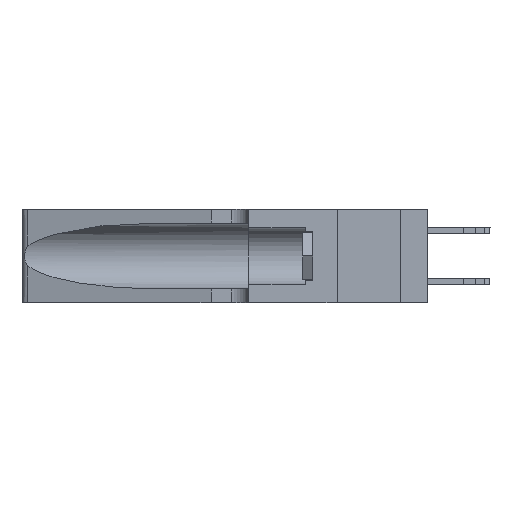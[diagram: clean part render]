
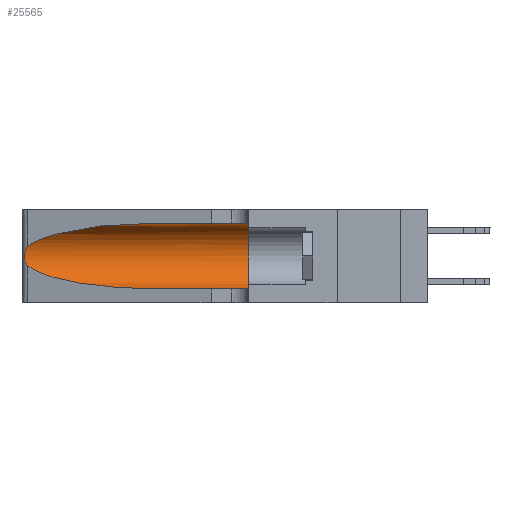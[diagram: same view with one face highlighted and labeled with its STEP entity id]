
A CAD part, left-side view. The second image highlights one B-rep face of the part: STEP entity #25565.
In plain terms, the highlighted cylindrical face has radius 3.308 mm (diameter 6.617 mm), a partial arc.
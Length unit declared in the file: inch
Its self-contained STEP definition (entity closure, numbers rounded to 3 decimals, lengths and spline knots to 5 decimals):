
#877 = CARTESIAN_POINT ( 'NONE',  ( 0.2373, 1.15595, 0.08982 ) ) ;
#1038 = ORIENTED_EDGE ( 'NONE', *, *, #34317, .F. ) ;
#1173 = DIRECTION ( 'NONE',  ( 0., 1., 0. ) ) ;
#3045 = CARTESIAN_POINT ( 'NONE',  ( 0.25787, 1.23484, 0.2124 ) ) ;
#4140 = DIRECTION ( 'NONE',  ( 0., -1., 0. ) ) ;
#4218 = DIRECTION ( 'NONE',  ( 0., 0., 1. ) ) ;
#6433 = B_SPLINE_CURVE_WITH_KNOTS ( 'NONE', 3,
 ( #35911, #26943, #24569, #3045, #27586, #21166, #18249, #9301, #9547, #6499, #30630, #33368, #12168, #15463 ),
 .UNSPECIFIED., .F., .F.,
 ( 4, 2, 2, 2, 2, 2, 4 ),
 ( 0., 0.00027, 0.00053, 0.00107, 0.0016, 0.00187, 0.00214 ),
 .UNSPECIFIED. ) ;
#6499 = CARTESIAN_POINT ( 'NONE',  ( 0.25856, 1.23593, 0.16098 ) ) ;
#6806 = CARTESIAN_POINT ( 'NONE',  ( 0.1305, 1.61858, 0.185 ) ) ;
#7029 = CYLINDRICAL_SURFACE ( 'NONE', #19081, 0.13025 ) ;
#9301 = CARTESIAN_POINT ( 'NONE',  ( 0.26075, 1.23896, 0.178 ) ) ;
#9453 = LINE ( 'NONE', #23665, #11319 ) ;
#9547 = CARTESIAN_POINT ( 'NONE',  ( 0.26017, 1.23833, 0.17102 ) ) ;
#10111 = CARTESIAN_POINT ( 'NONE',  ( 0.25487, 1.22718, 0.22369 ) ) ;
#10358 = CARTESIAN_POINT ( 'NONE',  ( 0.1305, 1.61858, 0.31525 ) ) ;
#11319 = VECTOR ( 'NONE', #17720, 39.37008 ) ;
#12168 = CARTESIAN_POINT ( 'NONE',  ( 0.25555, 1.22993, 0.14849 ) ) ;
#12415 = VECTOR ( 'NONE', #4140, 39.37008 ) ;
#12781 = CARTESIAN_POINT ( 'NONE',  ( 0.25487, 1.22718, 0.14631 ) ) ;
#13855 = CARTESIAN_POINT ( 'NONE',  ( 0.1305, 0.35, 0.05475 ) ) ;
#14553 = VERTEX_POINT ( 'NONE', #13855 ) ;
#15391 = AXIS2_PLACEMENT_3D ( 'NONE', #28091, #1173, #4218 ) ;
#15392 = EDGE_LOOP ( 'NONE', ( #38786, #21046, #20646, #25546, #38464, #1038 ) ) ;
#15463 = CARTESIAN_POINT ( 'NONE',  ( 0.25487, 1.22718, 0.14631 ) ) ;
#16828 = CARTESIAN_POINT ( 'NONE',  ( 0.1305, 0.72297, 0.31525 ) ) ;
#17142 = VERTEX_POINT ( 'NONE', #16828 ) ;
#17720 = DIRECTION ( 'NONE',  ( 0., -1., 0. ) ) ;
#18249 = CARTESIAN_POINT ( 'NONE',  ( 0.26075, 1.23896, 0.19203 ) ) ;
#19081 = AXIS2_PLACEMENT_3D ( 'NONE', #6806, #36607, #30418 ) ;
#20246 = FACE_OUTER_BOUND ( 'NONE', #15392, .T. ) ;
#20470 =( BOUNDED_CURVE ( )  B_SPLINE_CURVE ( 3, ( #12781, #877, #34147, #31241 ),
 .UNSPECIFIED., .F., .T. ) 
 B_SPLINE_CURVE_WITH_KNOTS ( ( 4, 4 ),
 ( 3.44316, 4.71239 ),
 .UNSPECIFIED. ) 
 CURVE ( )  GEOMETRIC_REPRESENTATION_ITEM ( )  RATIONAL_B_SPLINE_CURVE ( ( 1., 0.87, 0.87, 1. ) ) 
 REPRESENTATION_ITEM ( '' )  );
#20497 = EDGE_CURVE ( 'NONE', #17142, #31405, #26970, .T. ) ;
#20646 = ORIENTED_EDGE ( 'NONE', *, *, #33541, .T. ) ;
#21046 = ORIENTED_EDGE ( 'NONE', *, *, #36292, .T. ) ;
#21166 = CARTESIAN_POINT ( 'NONE',  ( 0.26018, 1.23835, 0.19895 ) ) ;
#22919 = CARTESIAN_POINT ( 'NONE',  ( 0.1305, 0.72297, 0.05475 ) ) ;
#23665 = CARTESIAN_POINT ( 'NONE',  ( 0.1305, 1.61858, 0.05475 ) ) ;
#23750 = LINE ( 'NONE', #10358, #12415 ) ;
#23792 = CIRCLE ( 'NONE', #15391, 0.13025 ) ;
#24172 = EDGE_CURVE ( 'NONE', #38237, #14553, #9453, .T. ) ;
#24569 = CARTESIAN_POINT ( 'NONE',  ( 0.25639, 1.23184, 0.21858 ) ) ;
#25546 = ORIENTED_EDGE ( 'NONE', *, *, #24172, .T. ) ;
#25565 = ADVANCED_FACE ( 'NONE', ( #20246 ), #7029, .F. ) ;
#26818 = CARTESIAN_POINT ( 'NONE',  ( 0.1305, 0.35, 0.31525 ) ) ;
#26943 = CARTESIAN_POINT ( 'NONE',  ( 0.25555, 1.22994, 0.2215 ) ) ;
#26970 =( BOUNDED_CURVE ( )  B_SPLINE_CURVE ( 3, ( #33704, #31198, #28147, #10111 ),
 .UNSPECIFIED., .F., .F. ) 
 B_SPLINE_CURVE_WITH_KNOTS ( ( 4, 4 ),
 ( 1.5708, 2.84003 ),
 .UNSPECIFIED. ) 
 CURVE ( )  GEOMETRIC_REPRESENTATION_ITEM ( )  RATIONAL_B_SPLINE_CURVE ( ( 1., 0.87, 0.87, 1. ) ) 
 REPRESENTATION_ITEM ( '' )  );
#27586 = CARTESIAN_POINT ( 'NONE',  ( 0.25854, 1.2359, 0.20912 ) ) ;
#28091 = CARTESIAN_POINT ( 'NONE',  ( 0.1305, 0.35, 0.185 ) ) ;
#28147 = CARTESIAN_POINT ( 'NONE',  ( 0.2373, 1.15595, 0.28018 ) ) ;
#28174 = VERTEX_POINT ( 'NONE', #32413 ) ;
#30418 = DIRECTION ( 'NONE',  ( 0., 0., -1. ) ) ;
#30523 = EDGE_CURVE ( 'NONE', #36168, #14553, #23792, .T. ) ;
#30630 = CARTESIAN_POINT ( 'NONE',  ( 0.25789, 1.23486, 0.15765 ) ) ;
#31198 = CARTESIAN_POINT ( 'NONE',  ( 0.18966, 0.96281, 0.31525 ) ) ;
#31241 = CARTESIAN_POINT ( 'NONE',  ( 0.1305, 0.72297, 0.05475 ) ) ;
#31405 = VERTEX_POINT ( 'NONE', #38350 ) ;
#32413 = CARTESIAN_POINT ( 'NONE',  ( 0.25487, 1.22718, 0.14631 ) ) ;
#33368 = CARTESIAN_POINT ( 'NONE',  ( 0.25639, 1.23186, 0.15144 ) ) ;
#33541 = EDGE_CURVE ( 'NONE', #28174, #38237, #20470, .T. ) ;
#33704 = CARTESIAN_POINT ( 'NONE',  ( 0.1305, 0.72297, 0.31525 ) ) ;
#34147 = CARTESIAN_POINT ( 'NONE',  ( 0.18966, 0.96281, 0.05475 ) ) ;
#34317 = EDGE_CURVE ( 'NONE', #17142, #36168, #23750, .T. ) ;
#35911 = CARTESIAN_POINT ( 'NONE',  ( 0.25487, 1.22718, 0.22369 ) ) ;
#36168 = VERTEX_POINT ( 'NONE', #26818 ) ;
#36292 = EDGE_CURVE ( 'NONE', #31405, #28174, #6433, .T. ) ;
#36607 = DIRECTION ( 'NONE',  ( 0., -1., 0. ) ) ;
#38237 = VERTEX_POINT ( 'NONE', #22919 ) ;
#38350 = CARTESIAN_POINT ( 'NONE',  ( 0.25487, 1.22718, 0.22369 ) ) ;
#38464 = ORIENTED_EDGE ( 'NONE', *, *, #30523, .F. ) ;
#38786 = ORIENTED_EDGE ( 'NONE', *, *, #20497, .T. ) ;
